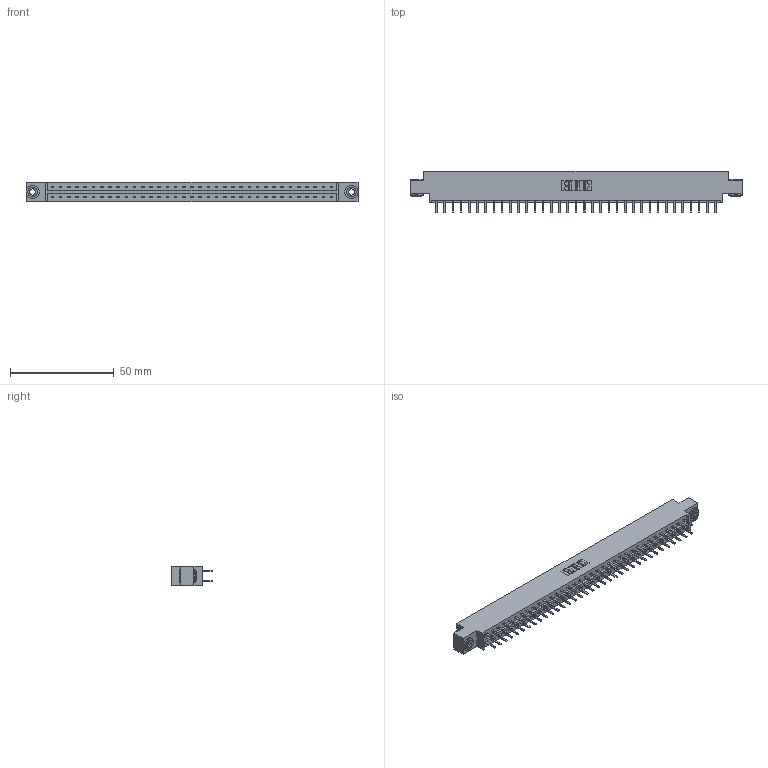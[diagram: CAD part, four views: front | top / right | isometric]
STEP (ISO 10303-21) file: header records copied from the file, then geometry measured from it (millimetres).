
FILE_DESCRIPTION (( 'STEP AP203' ), '1' );
FILE_NAME ('333-070-520-803.STEP', '2018-08-04T14:14:09', ( '' ), ( '' ), 'SwSTEP 2.0', 'SolidWorks 2016', '' );
FILE_SCHEMA (( 'CONFIG_CONTROL_DESIGN' ));
Length unit declared in the file: inch
Products named in the file (4): 333-070-520-803; 333 Part_Offset - .156 Dia - TH; 345-292-001_345-293-120; 345-250-002_345-250-002-102
Assembly tree (73 placements, depth 2):
  333-070-520-803
    333 Part_Offset - .156 Dia - TH
    345-292-001_345-293-120  x70
    345-250-002_345-250-002-102  x2
Bounding box: 160.22 x 20.02 x 9.4 mm (x, y, z)
Volume: 16053.2 mm3; surface area: 19263.9 mm2
Topology: 73 solids, 73 shells, 4076 faces, 11809 edges, 7682 vertices
Faces by surface type: plane 2744, cylinder 1324, cone 8
Entity records: 24318 total; most frequent: CARTESIAN_POINT 4029, ORIENTED_EDGE 3946, DIRECTION 3475, EDGE_CURVE 1973, VECTOR 1817, LINE 1817, VERTEX_POINT 1310, AXIS2_PLACEMENT_3D 829
